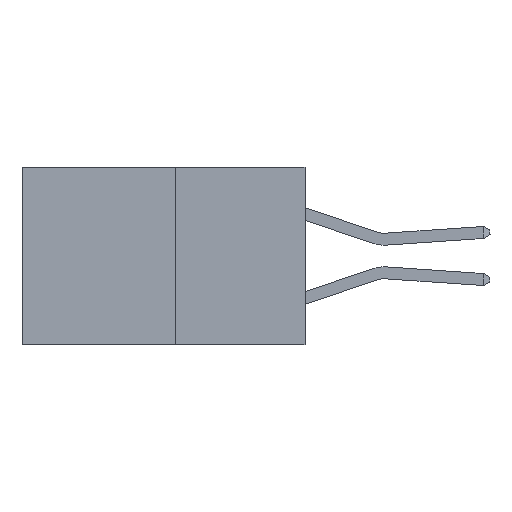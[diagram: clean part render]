
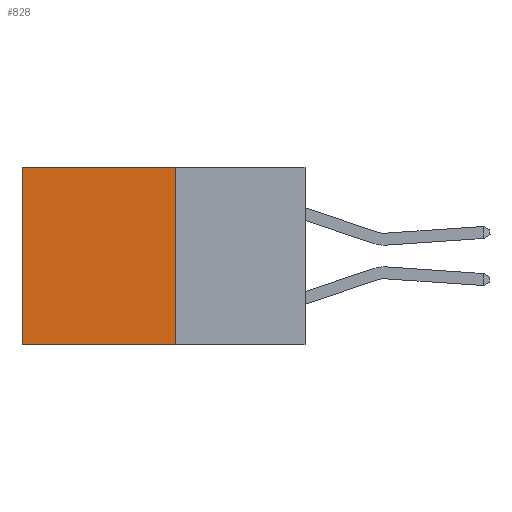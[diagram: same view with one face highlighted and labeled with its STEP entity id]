
A CAD part, left-side view. The second image highlights one B-rep face of the part: STEP entity #828.
In plain terms, the highlighted planar face has unit normal (-1, 0, 0).
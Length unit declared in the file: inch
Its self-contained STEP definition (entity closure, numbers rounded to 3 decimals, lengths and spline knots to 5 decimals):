
#482 = CARTESIAN_POINT ( 'NONE',  ( 0.277, 0.27, -0.37 ) ) ;
#828 = ADVANCED_FACE ( 'NONE', ( #837 ), #6742, .F. ) ;
#837 = FACE_OUTER_BOUND ( 'NONE', #12648, .T. ) ;
#997 = DIRECTION ( 'NONE',  ( 0., 0., -1. ) ) ;
#1530 = LINE ( 'NONE', #2308, #1853 ) ;
#1853 = VECTOR ( 'NONE', #2549, 39.37008 ) ;
#2308 = CARTESIAN_POINT ( 'NONE',  ( 0.277, 0.27, -0.37 ) ) ;
#2324 = ORIENTED_EDGE ( 'NONE', *, *, #9077, .T. ) ;
#2549 = DIRECTION ( 'NONE',  ( 0., 1., 0. ) ) ;
#2962 = LINE ( 'NONE', #10141, #10531 ) ;
#3005 = ORIENTED_EDGE ( 'NONE', *, *, #5914, .F. ) ;
#3315 = LINE ( 'NONE', #9737, #11535 ) ;
#3631 = ORIENTED_EDGE ( 'NONE', *, *, #3739, .F. ) ;
#3739 = EDGE_CURVE ( 'NONE', #12909, #7453, #11260, .T. ) ;
#3951 = ORIENTED_EDGE ( 'NONE', *, *, #4657, .T. ) ;
#4657 = EDGE_CURVE ( 'NONE', #12909, #8737, #3315, .T. ) ;
#4968 = DIRECTION ( 'NONE',  ( 1., 0., 0. ) ) ;
#5551 = CARTESIAN_POINT ( 'NONE',  ( 0.277, 0.59, 0. ) ) ;
#5914 = EDGE_CURVE ( 'NONE', #7453, #10973, #1530, .T. ) ;
#6742 = PLANE ( 'NONE',  #12014 ) ;
#7453 = VERTEX_POINT ( 'NONE', #482 ) ;
#8047 = DIRECTION ( 'NONE',  ( 0., 0., -1. ) ) ;
#8474 = VECTOR ( 'NONE', #10907, 39.37008 ) ;
#8737 = VERTEX_POINT ( 'NONE', #5551 ) ;
#9077 = EDGE_CURVE ( 'NONE', #8737, #10973, #2962, .T. ) ;
#9735 = DIRECTION ( 'NONE',  ( 0., 1., 0. ) ) ;
#9737 = CARTESIAN_POINT ( 'NONE',  ( 0.277, 0.27, 0. ) ) ;
#9966 = CARTESIAN_POINT ( 'NONE',  ( 0.277, 0.27, -0.37 ) ) ;
#10141 = CARTESIAN_POINT ( 'NONE',  ( 0.277, 0.59, -0.37 ) ) ;
#10531 = VECTOR ( 'NONE', #8047, 39.37008 ) ;
#10907 = DIRECTION ( 'NONE',  ( 0., 0., -1. ) ) ;
#10973 = VERTEX_POINT ( 'NONE', #12872 ) ;
#11260 = LINE ( 'NONE', #9966, #8474 ) ;
#11535 = VECTOR ( 'NONE', #9735, 39.37008 ) ;
#12014 = AXIS2_PLACEMENT_3D ( 'NONE', #12697, #4968, #997 ) ;
#12598 = CARTESIAN_POINT ( 'NONE',  ( 0.277, 0.27, 0. ) ) ;
#12648 = EDGE_LOOP ( 'NONE', ( #2324, #3005, #3631, #3951 ) ) ;
#12697 = CARTESIAN_POINT ( 'NONE',  ( 0.277, 0.27, -0.37 ) ) ;
#12872 = CARTESIAN_POINT ( 'NONE',  ( 0.277, 0.59, -0.37 ) ) ;
#12909 = VERTEX_POINT ( 'NONE', #12598 ) ;
